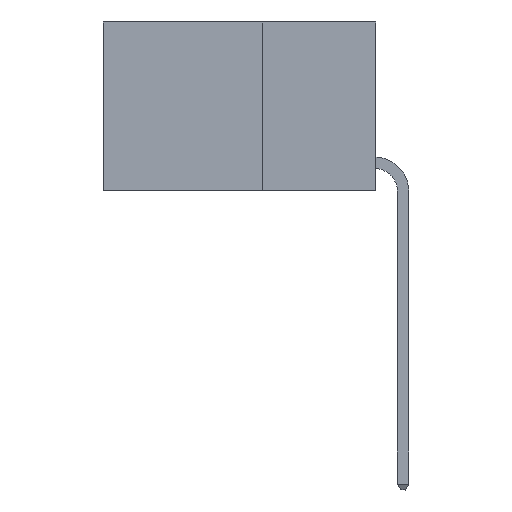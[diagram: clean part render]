
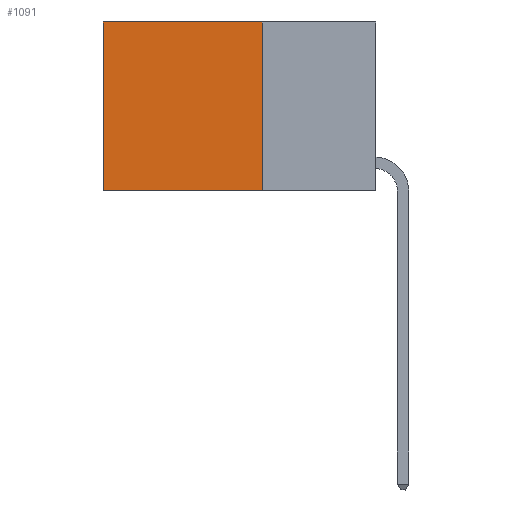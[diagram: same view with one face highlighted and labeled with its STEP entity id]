
A CAD part, left-side view. The second image highlights one B-rep face of the part: STEP entity #1091.
In plain terms, the highlighted planar face has unit normal (-1, 0, 0).
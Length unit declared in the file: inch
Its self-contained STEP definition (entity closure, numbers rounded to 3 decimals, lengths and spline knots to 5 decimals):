
#682 = VECTOR ( 'NONE', #4412, 39.37008 ) ;
#761 = CARTESIAN_POINT ( 'NONE',  ( 0.2625, 0.25, 0. ) ) ;
#893 = CARTESIAN_POINT ( 'NONE',  ( 0.2625, 0.25, -0.37 ) ) ;
#1080 = CARTESIAN_POINT ( 'NONE',  ( 0.2625, 0.6, 0. ) ) ;
#1091 = ADVANCED_FACE ( 'NONE', ( #4107 ), #2082, .F. ) ;
#1301 = VERTEX_POINT ( 'NONE', #7980 ) ;
#1359 = VERTEX_POINT ( 'NONE', #1080 ) ;
#2082 = PLANE ( 'NONE',  #9078 ) ;
#2194 = VECTOR ( 'NONE', #11381, 39.37008 ) ;
#2402 = CARTESIAN_POINT ( 'NONE',  ( 0.2625, 0.25, 0. ) ) ;
#2907 = ORIENTED_EDGE ( 'NONE', *, *, #10121, .T. ) ;
#3199 = ORIENTED_EDGE ( 'NONE', *, *, #10899, .F. ) ;
#3342 = EDGE_CURVE ( 'NONE', #8561, #8630, #4213, .T. ) ;
#3472 = ORIENTED_EDGE ( 'NONE', *, *, #9593, .T. ) ;
#4107 = FACE_OUTER_BOUND ( 'NONE', #8069, .T. ) ;
#4144 = CARTESIAN_POINT ( 'NONE',  ( 0.2625, 0.25, 0. ) ) ;
#4213 = LINE ( 'NONE', #8101, #8740 ) ;
#4412 = DIRECTION ( 'NONE',  ( 0., 1., 0. ) ) ;
#4937 = LINE ( 'NONE', #4144, #11531 ) ;
#5367 = CARTESIAN_POINT ( 'NONE',  ( 0.2625, 0.6, 0. ) ) ;
#5462 = LINE ( 'NONE', #10580, #682 ) ;
#5663 = DIRECTION ( 'NONE',  ( 1., 0., 0. ) ) ;
#6050 = DIRECTION ( 'NONE',  ( 0., 0., -1. ) ) ;
#6207 = LINE ( 'NONE', #5367, #2194 ) ;
#6906 = DIRECTION ( 'NONE',  ( 0., 1., 0. ) ) ;
#7883 = DIRECTION ( 'NONE',  ( 0., 0., -1. ) ) ;
#7980 = CARTESIAN_POINT ( 'NONE',  ( 0.2625, 0.6, -0.37 ) ) ;
#8069 = EDGE_LOOP ( 'NONE', ( #2907, #3199, #11072, #3472 ) ) ;
#8101 = CARTESIAN_POINT ( 'NONE',  ( 0.2625, 0.25, 0. ) ) ;
#8561 = VERTEX_POINT ( 'NONE', #761 ) ;
#8630 = VERTEX_POINT ( 'NONE', #893 ) ;
#8740 = VECTOR ( 'NONE', #7883, 39.37008 ) ;
#9078 = AXIS2_PLACEMENT_3D ( 'NONE', #2402, #5663, #6050 ) ;
#9593 = EDGE_CURVE ( 'NONE', #8561, #1359, #4937, .T. ) ;
#10121 = EDGE_CURVE ( 'NONE', #1359, #1301, #6207, .T. ) ;
#10580 = CARTESIAN_POINT ( 'NONE',  ( 0.2625, 0.25, -0.37 ) ) ;
#10899 = EDGE_CURVE ( 'NONE', #8630, #1301, #5462, .T. ) ;
#11072 = ORIENTED_EDGE ( 'NONE', *, *, #3342, .F. ) ;
#11381 = DIRECTION ( 'NONE',  ( 0., 0., -1. ) ) ;
#11531 = VECTOR ( 'NONE', #6906, 39.37008 ) ;
